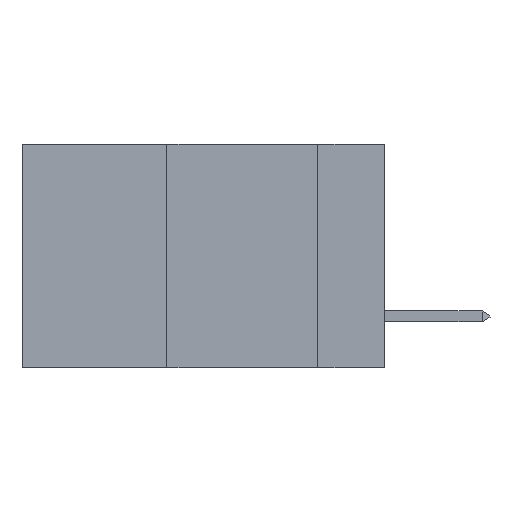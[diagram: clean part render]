
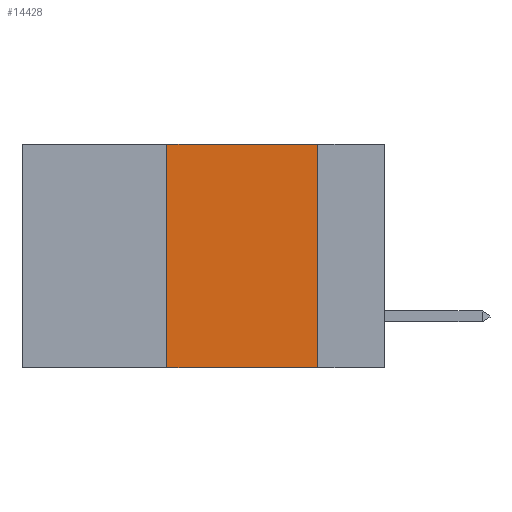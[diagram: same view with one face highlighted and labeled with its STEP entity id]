
A CAD part, left-side view. The second image highlights one B-rep face of the part: STEP entity #14428.
In plain terms, the highlighted planar face has unit normal (-1, 0, 0).
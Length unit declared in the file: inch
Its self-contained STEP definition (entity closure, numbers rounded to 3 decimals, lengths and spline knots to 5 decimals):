
#2749 = ORIENTED_EDGE ( 'NONE', *, *, #27125, .F. ) ;
#4500 = VECTOR ( 'NONE', #32413, 39.37008 ) ;
#4668 = VECTOR ( 'NONE', #6787, 39.37008 ) ;
#5185 = VERTEX_POINT ( 'NONE', #30442 ) ;
#5366 = LINE ( 'NONE', #16574, #4500 ) ;
#6787 = DIRECTION ( 'NONE',  ( 0., -1., 0. ) ) ;
#6886 = DIRECTION ( 'NONE',  ( 0., -1., 0. ) ) ;
#7089 = CARTESIAN_POINT ( 'NONE',  ( 0., 0.36, 0. ) ) ;
#7122 = CARTESIAN_POINT ( 'NONE',  ( 0., 0.36, 0. ) ) ;
#7536 = CARTESIAN_POINT ( 'NONE',  ( 0., 0.11, -0.37 ) ) ;
#9494 = EDGE_CURVE ( 'NONE', #12659, #5185, #16876, .T. ) ;
#9934 = VERTEX_POINT ( 'NONE', #33405 ) ;
#11618 = VERTEX_POINT ( 'NONE', #7536 ) ;
#12009 = LINE ( 'NONE', #12210, #4668 ) ;
#12045 = EDGE_CURVE ( 'NONE', #9934, #11618, #12009, .T. ) ;
#12210 = CARTESIAN_POINT ( 'NONE',  ( 0., 0.6, -0.37 ) ) ;
#12659 = VERTEX_POINT ( 'NONE', #7089 ) ;
#13206 = FACE_OUTER_BOUND ( 'NONE', #13918, .T. ) ;
#13918 = EDGE_LOOP ( 'NONE', ( #26941, #14059, #2749, #29659 ) ) ;
#14059 = ORIENTED_EDGE ( 'NONE', *, *, #9494, .F. ) ;
#14428 = ADVANCED_FACE ( 'NONE', ( #13206 ), #28658, .F. ) ;
#14677 = EDGE_CURVE ( 'NONE', #5185, #11618, #5366, .T. ) ;
#15145 = CARTESIAN_POINT ( 'NONE',  ( 0., 0.6, 0. ) ) ;
#15551 = CARTESIAN_POINT ( 'NONE',  ( 0., 0.6, 0. ) ) ;
#16574 = CARTESIAN_POINT ( 'NONE',  ( 0., 0.11, 0. ) ) ;
#16876 = LINE ( 'NONE', #15145, #23154 ) ;
#17913 = AXIS2_PLACEMENT_3D ( 'NONE', #15551, #34040, #18213 ) ;
#18213 = DIRECTION ( 'NONE',  ( 0., 0., -1. ) ) ;
#20865 = DIRECTION ( 'NONE',  ( 0., 0., 1. ) ) ;
#23154 = VECTOR ( 'NONE', #6886, 39.37008 ) ;
#26941 = ORIENTED_EDGE ( 'NONE', *, *, #14677, .F. ) ;
#27125 = EDGE_CURVE ( 'NONE', #9934, #12659, #27384, .T. ) ;
#27384 = LINE ( 'NONE', #7122, #31884 ) ;
#28658 = PLANE ( 'NONE',  #17913 ) ;
#29659 = ORIENTED_EDGE ( 'NONE', *, *, #12045, .T. ) ;
#30442 = CARTESIAN_POINT ( 'NONE',  ( 0., 0.11, 0. ) ) ;
#31884 = VECTOR ( 'NONE', #20865, 39.37008 ) ;
#32413 = DIRECTION ( 'NONE',  ( 0., 0., -1. ) ) ;
#33405 = CARTESIAN_POINT ( 'NONE',  ( 0., 0.36, -0.37 ) ) ;
#34040 = DIRECTION ( 'NONE',  ( 1., 0., 0. ) ) ;
